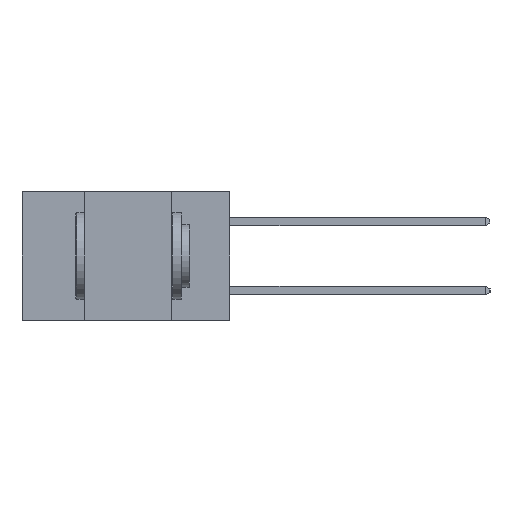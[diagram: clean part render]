
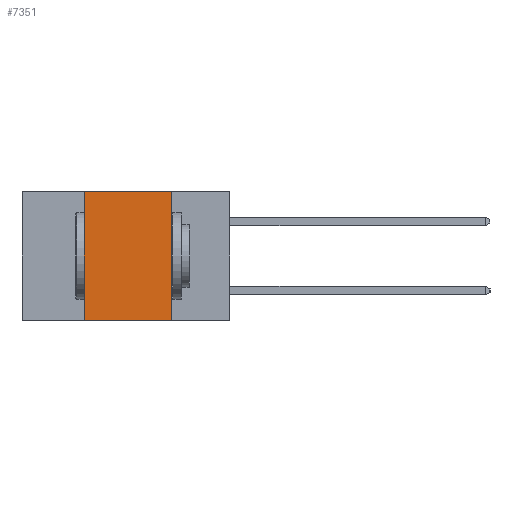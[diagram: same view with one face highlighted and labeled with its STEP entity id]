
A CAD part, left-side view. The second image highlights one B-rep face of the part: STEP entity #7351.
In plain terms, the highlighted planar face has unit normal (-1, 0, 0).
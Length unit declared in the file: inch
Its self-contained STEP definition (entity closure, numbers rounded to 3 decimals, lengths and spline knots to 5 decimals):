
#311 = AXIS2_PLACEMENT_3D ( 'NONE', #9853, #9820, #9762 ) ;
#856 = VECTOR ( 'NONE', #13971, 39.37008 ) ;
#913 = EDGE_CURVE ( 'NONE', #10355, #15455, #14711, .T. ) ;
#2225 = CARTESIAN_POINT ( 'NONE',  ( 0., 0.17, -0.37 ) ) ;
#2769 = FACE_OUTER_BOUND ( 'NONE', #7033, .T. ) ;
#3182 = DIRECTION ( 'NONE',  ( 0., 0., -1. ) ) ;
#4825 = CARTESIAN_POINT ( 'NONE',  ( 0., 0.42, -0.37 ) ) ;
#7033 = EDGE_LOOP ( 'NONE', ( #15920, #19213, #14394, #23082 ) ) ;
#7351 = ADVANCED_FACE ( 'NONE', ( #2769 ), #9939, .F. ) ;
#9365 = VECTOR ( 'NONE', #12689, 39.37008 ) ;
#9762 = DIRECTION ( 'NONE',  ( 0., 0., -1. ) ) ;
#9820 = DIRECTION ( 'NONE',  ( 1., 0., 0. ) ) ;
#9853 = CARTESIAN_POINT ( 'NONE',  ( 0., 0.6, 0. ) ) ;
#9939 = PLANE ( 'NONE',  #311 ) ;
#10355 = VERTEX_POINT ( 'NONE', #19506 ) ;
#11691 = CARTESIAN_POINT ( 'NONE',  ( 0., 0.17, 0. ) ) ;
#12689 = DIRECTION ( 'NONE',  ( 0., 0., 1. ) ) ;
#12771 = CARTESIAN_POINT ( 'NONE',  ( 0., 0.6, 0. ) ) ;
#13971 = DIRECTION ( 'NONE',  ( 0., -1., 0. ) ) ;
#14394 = ORIENTED_EDGE ( 'NONE', *, *, #913, .F. ) ;
#14557 = CARTESIAN_POINT ( 'NONE',  ( 0., 0.42, 0. ) ) ;
#14711 = LINE ( 'NONE', #4825, #9365 ) ;
#15455 = VERTEX_POINT ( 'NONE', #14557 ) ;
#15920 = ORIENTED_EDGE ( 'NONE', *, *, #24613, .F. ) ;
#15939 = LINE ( 'NONE', #17232, #20488 ) ;
#16675 = LINE ( 'NONE', #12771, #21173 ) ;
#16949 = LINE ( 'NONE', #19840, #856 ) ;
#17232 = CARTESIAN_POINT ( 'NONE',  ( 0., 0.17, -0.37 ) ) ;
#17246 = EDGE_CURVE ( 'NONE', #10355, #24292, #16949, .T. ) ;
#18543 = DIRECTION ( 'NONE',  ( 0., -1., 0. ) ) ;
#19213 = ORIENTED_EDGE ( 'NONE', *, *, #22554, .F. ) ;
#19506 = CARTESIAN_POINT ( 'NONE',  ( 0., 0.42, -0.37 ) ) ;
#19725 = VERTEX_POINT ( 'NONE', #11691 ) ;
#19840 = CARTESIAN_POINT ( 'NONE',  ( 0., 0.6, -0.37 ) ) ;
#20488 = VECTOR ( 'NONE', #3182, 39.37008 ) ;
#21173 = VECTOR ( 'NONE', #18543, 39.37008 ) ;
#22554 = EDGE_CURVE ( 'NONE', #15455, #19725, #16675, .T. ) ;
#23082 = ORIENTED_EDGE ( 'NONE', *, *, #17246, .T. ) ;
#24292 = VERTEX_POINT ( 'NONE', #2225 ) ;
#24613 = EDGE_CURVE ( 'NONE', #19725, #24292, #15939, .T. ) ;
